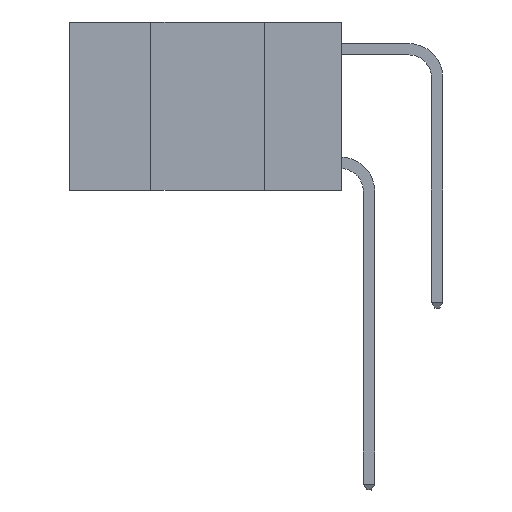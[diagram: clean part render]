
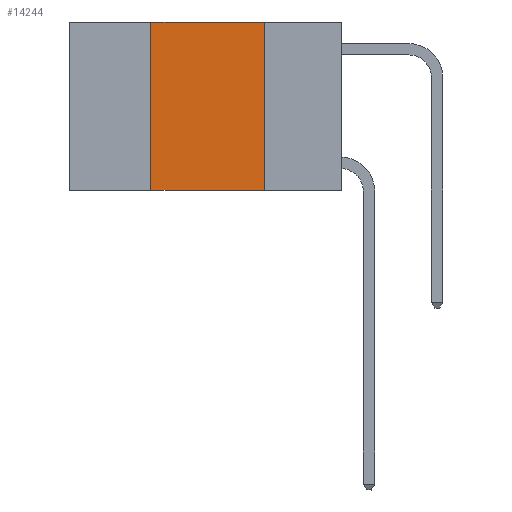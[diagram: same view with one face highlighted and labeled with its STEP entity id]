
A CAD part, left-side view. The second image highlights one B-rep face of the part: STEP entity #14244.
In plain terms, the highlighted planar face has unit normal (-1, 0, 0).
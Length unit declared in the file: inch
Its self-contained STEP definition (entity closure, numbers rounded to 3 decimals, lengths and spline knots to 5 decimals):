
#558 = CARTESIAN_POINT ( 'NONE',  ( 0., 0.17, 0. ) ) ;
#1252 = DIRECTION ( 'NONE',  ( 0., 0., 1. ) ) ;
#1767 = EDGE_CURVE ( 'NONE', #7235, #12802, #13848, .T. ) ;
#3227 = EDGE_CURVE ( 'NONE', #7235, #19088, #5686, .T. ) ;
#3379 = ORIENTED_EDGE ( 'NONE', *, *, #1767, .T. ) ;
#3726 = CARTESIAN_POINT ( 'NONE',  ( 0., 0.17, -0.37 ) ) ;
#4453 = EDGE_CURVE ( 'NONE', #19088, #10134, #10583, .T. ) ;
#5686 = LINE ( 'NONE', #15903, #10089 ) ;
#6203 = DIRECTION ( 'NONE',  ( 0., -1., 0. ) ) ;
#7108 = DIRECTION ( 'NONE',  ( 0., 0., -1. ) ) ;
#7235 = VERTEX_POINT ( 'NONE', #12635 ) ;
#8397 = CARTESIAN_POINT ( 'NONE',  ( 0., 0.6, -0.37 ) ) ;
#8470 = DIRECTION ( 'NONE',  ( 0., -1., 0. ) ) ;
#8952 = CARTESIAN_POINT ( 'NONE',  ( 0., 0.17, 0. ) ) ;
#9101 = DIRECTION ( 'NONE',  ( 0., 0., -1. ) ) ;
#9803 = DIRECTION ( 'NONE',  ( 1., 0., 0. ) ) ;
#10071 = VECTOR ( 'NONE', #6203, 39.37008 ) ;
#10089 = VECTOR ( 'NONE', #1252, 39.37008 ) ;
#10134 = VERTEX_POINT ( 'NONE', #8952 ) ;
#10583 = LINE ( 'NONE', #19045, #10071 ) ;
#10788 = VECTOR ( 'NONE', #8470, 39.37008 ) ;
#12635 = CARTESIAN_POINT ( 'NONE',  ( 0., 0.42, -0.37 ) ) ;
#12802 = VERTEX_POINT ( 'NONE', #3726 ) ;
#13436 = VECTOR ( 'NONE', #7108, 39.37008 ) ;
#13757 = FACE_OUTER_BOUND ( 'NONE', #18337, .T. ) ;
#13848 = LINE ( 'NONE', #8397, #10788 ) ;
#14244 = ADVANCED_FACE ( 'NONE', ( #13757 ), #19508, .F. ) ;
#14564 = ORIENTED_EDGE ( 'NONE', *, *, #17611, .F. ) ;
#15428 = AXIS2_PLACEMENT_3D ( 'NONE', #19581, #9803, #9101 ) ;
#15903 = CARTESIAN_POINT ( 'NONE',  ( 0., 0.42, 0. ) ) ;
#17611 = EDGE_CURVE ( 'NONE', #10134, #12802, #19827, .T. ) ;
#17722 = ORIENTED_EDGE ( 'NONE', *, *, #4453, .F. ) ;
#18337 = EDGE_LOOP ( 'NONE', ( #14564, #17722, #20224, #3379 ) ) ;
#18495 = CARTESIAN_POINT ( 'NONE',  ( 0., 0.42, 0. ) ) ;
#19045 = CARTESIAN_POINT ( 'NONE',  ( 0., 0.6, 0. ) ) ;
#19088 = VERTEX_POINT ( 'NONE', #18495 ) ;
#19508 = PLANE ( 'NONE',  #15428 ) ;
#19581 = CARTESIAN_POINT ( 'NONE',  ( 0., 0.6, 0. ) ) ;
#19827 = LINE ( 'NONE', #558, #13436 ) ;
#20224 = ORIENTED_EDGE ( 'NONE', *, *, #3227, .F. ) ;
